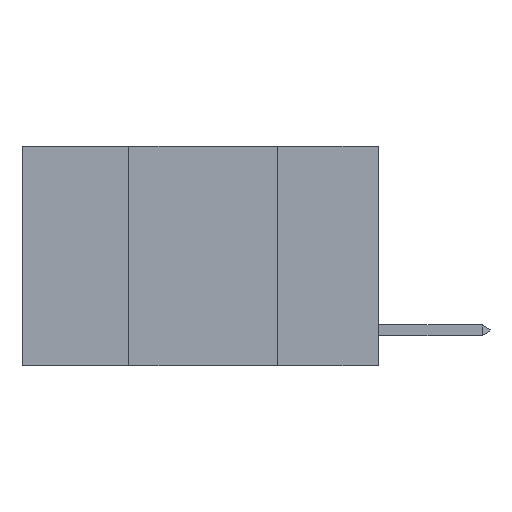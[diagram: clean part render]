
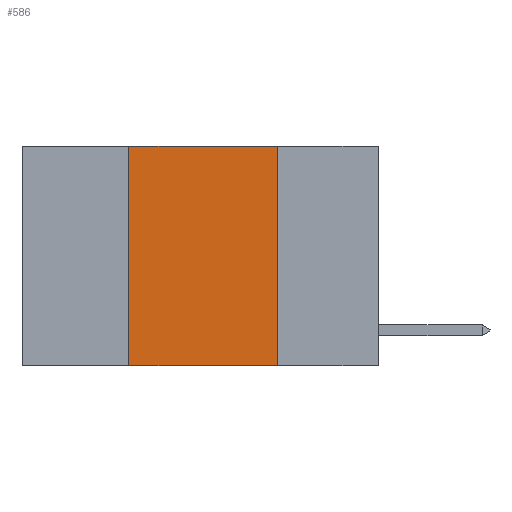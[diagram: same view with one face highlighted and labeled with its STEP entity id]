
A CAD part, left-side view. The second image highlights one B-rep face of the part: STEP entity #586.
In plain terms, the highlighted planar face has unit normal (-1, 0, 0).
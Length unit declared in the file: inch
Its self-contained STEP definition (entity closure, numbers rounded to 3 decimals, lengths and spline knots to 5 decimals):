
#508 = CARTESIAN_POINT ( 'NONE',  ( 0., 0.6, 0. ) ) ;
#586 = ADVANCED_FACE ( 'NONE', ( #4128 ), #18991, .F. ) ;
#1323 = VERTEX_POINT ( 'NONE', #19483 ) ;
#1739 = CARTESIAN_POINT ( 'NONE',  ( 0., 0.42, 0. ) ) ;
#4128 = FACE_OUTER_BOUND ( 'NONE', #23392, .T. ) ;
#4641 = CARTESIAN_POINT ( 'NONE',  ( 0., 0.42, -0.37 ) ) ;
#5200 = EDGE_CURVE ( 'NONE', #6531, #13051, #22287, .T. ) ;
#5848 = VERTEX_POINT ( 'NONE', #4641 ) ;
#6237 = AXIS2_PLACEMENT_3D ( 'NONE', #508, #21557, #11907 ) ;
#6531 = VERTEX_POINT ( 'NONE', #17269 ) ;
#7435 = EDGE_CURVE ( 'NONE', #5848, #6531, #17374, .T. ) ;
#7649 = ORIENTED_EDGE ( 'NONE', *, *, #5200, .F. ) ;
#8299 = CARTESIAN_POINT ( 'NONE',  ( 0., 0.6, 0. ) ) ;
#8641 = EDGE_CURVE ( 'NONE', #13051, #1323, #21245, .T. ) ;
#9137 = DIRECTION ( 'NONE',  ( 0., 0., 1. ) ) ;
#11503 = DIRECTION ( 'NONE',  ( 0., -1., 0. ) ) ;
#11907 = DIRECTION ( 'NONE',  ( 0., 0., -1. ) ) ;
#12037 = VECTOR ( 'NONE', #9137, 39.37008 ) ;
#13051 = VERTEX_POINT ( 'NONE', #23094 ) ;
#13492 = VECTOR ( 'NONE', #11503, 39.37008 ) ;
#13936 = VECTOR ( 'NONE', #20821, 39.37008 ) ;
#15013 = CARTESIAN_POINT ( 'NONE',  ( 0., 0.6, -0.37 ) ) ;
#16479 = DIRECTION ( 'NONE',  ( 0., 0., -1. ) ) ;
#17103 = VECTOR ( 'NONE', #16479, 39.37008 ) ;
#17269 = CARTESIAN_POINT ( 'NONE',  ( 0., 0.42, 0. ) ) ;
#17374 = LINE ( 'NONE', #1739, #12037 ) ;
#18277 = LINE ( 'NONE', #15013, #13492 ) ;
#18354 = CARTESIAN_POINT ( 'NONE',  ( 0., 0.17, 0. ) ) ;
#18991 = PLANE ( 'NONE',  #6237 ) ;
#19223 = ORIENTED_EDGE ( 'NONE', *, *, #22271, .T. ) ;
#19483 = CARTESIAN_POINT ( 'NONE',  ( 0., 0.17, -0.37 ) ) ;
#19549 = ORIENTED_EDGE ( 'NONE', *, *, #8641, .F. ) ;
#20809 = ORIENTED_EDGE ( 'NONE', *, *, #7435, .F. ) ;
#20821 = DIRECTION ( 'NONE',  ( 0., -1., 0. ) ) ;
#21245 = LINE ( 'NONE', #18354, #17103 ) ;
#21557 = DIRECTION ( 'NONE',  ( 1., 0., 0. ) ) ;
#22271 = EDGE_CURVE ( 'NONE', #5848, #1323, #18277, .T. ) ;
#22287 = LINE ( 'NONE', #8299, #13936 ) ;
#23094 = CARTESIAN_POINT ( 'NONE',  ( 0., 0.17, 0. ) ) ;
#23392 = EDGE_LOOP ( 'NONE', ( #19549, #7649, #20809, #19223 ) ) ;
